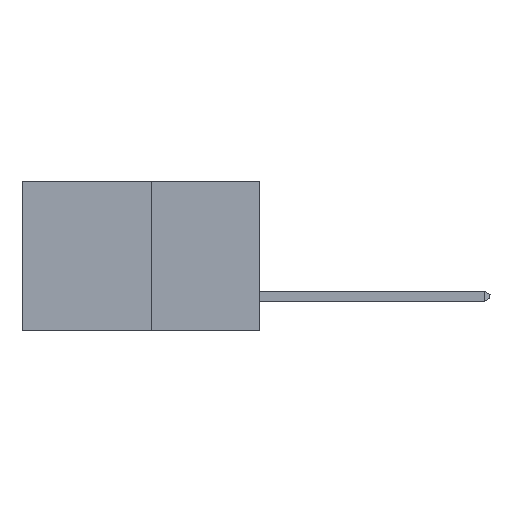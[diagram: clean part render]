
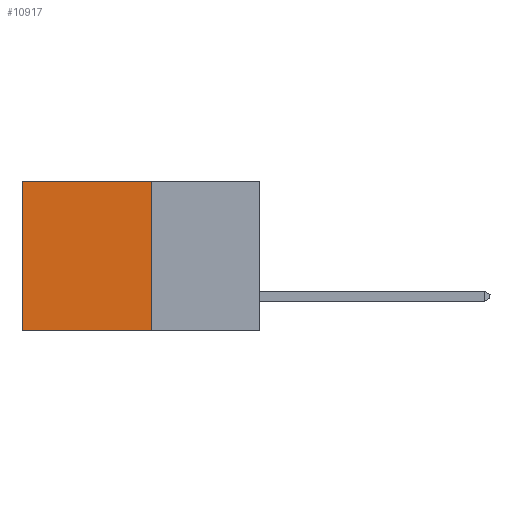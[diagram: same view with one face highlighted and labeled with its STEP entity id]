
A CAD part, left-side view. The second image highlights one B-rep face of the part: STEP entity #10917.
In plain terms, the highlighted planar face has unit normal (-1, 0, 0).
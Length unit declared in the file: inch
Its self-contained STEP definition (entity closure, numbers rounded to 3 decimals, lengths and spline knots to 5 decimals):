
#676 = EDGE_CURVE ( 'NONE', #6583, #10070, #5515, .T. ) ;
#762 = CARTESIAN_POINT ( 'NONE',  ( 0.277, 0.27, 0. ) ) ;
#1182 = DIRECTION ( 'NONE',  ( 0., 0., -1. ) ) ;
#1195 = ORIENTED_EDGE ( 'NONE', *, *, #676, .F. ) ;
#1271 = EDGE_CURVE ( 'NONE', #6583, #7665, #12351, .T. ) ;
#1290 = VECTOR ( 'NONE', #14383, 39.37008 ) ;
#1567 = CARTESIAN_POINT ( 'NONE',  ( 0.277, 0.59, 0. ) ) ;
#1625 = AXIS2_PLACEMENT_3D ( 'NONE', #15243, #8403, #1182 ) ;
#1984 = CARTESIAN_POINT ( 'NONE',  ( 0.277, 0.27, -0.37 ) ) ;
#2161 = LINE ( 'NONE', #12939, #14257 ) ;
#2253 = VECTOR ( 'NONE', #12042, 39.37008 ) ;
#2438 = CARTESIAN_POINT ( 'NONE',  ( 0.277, 0.59, -0.37 ) ) ;
#3572 = CARTESIAN_POINT ( 'NONE',  ( 0.277, 0.27, 0. ) ) ;
#4647 = LINE ( 'NONE', #12113, #1290 ) ;
#4787 = EDGE_LOOP ( 'NONE', ( #7700, #13098, #1195, #12960 ) ) ;
#5515 = LINE ( 'NONE', #14503, #2253 ) ;
#5862 = VECTOR ( 'NONE', #9073, 39.37008 ) ;
#6583 = VERTEX_POINT ( 'NONE', #3572 ) ;
#7665 = VERTEX_POINT ( 'NONE', #1567 ) ;
#7700 = ORIENTED_EDGE ( 'NONE', *, *, #13392, .T. ) ;
#8351 = DIRECTION ( 'NONE',  ( 0., 1., 0. ) ) ;
#8403 = DIRECTION ( 'NONE',  ( 1., 0., 0. ) ) ;
#9073 = DIRECTION ( 'NONE',  ( 0., 1., 0. ) ) ;
#10070 = VERTEX_POINT ( 'NONE', #1984 ) ;
#10861 = FACE_OUTER_BOUND ( 'NONE', #4787, .T. ) ;
#10886 = EDGE_CURVE ( 'NONE', #10070, #13913, #2161, .T. ) ;
#10917 = ADVANCED_FACE ( 'NONE', ( #10861 ), #14143, .F. ) ;
#12042 = DIRECTION ( 'NONE',  ( 0., 0., -1. ) ) ;
#12113 = CARTESIAN_POINT ( 'NONE',  ( 0.277, 0.59, -0.37 ) ) ;
#12351 = LINE ( 'NONE', #762, #5862 ) ;
#12939 = CARTESIAN_POINT ( 'NONE',  ( 0.277, 0.27, -0.37 ) ) ;
#12960 = ORIENTED_EDGE ( 'NONE', *, *, #1271, .T. ) ;
#13098 = ORIENTED_EDGE ( 'NONE', *, *, #10886, .F. ) ;
#13392 = EDGE_CURVE ( 'NONE', #7665, #13913, #4647, .T. ) ;
#13913 = VERTEX_POINT ( 'NONE', #2438 ) ;
#14143 = PLANE ( 'NONE',  #1625 ) ;
#14257 = VECTOR ( 'NONE', #8351, 39.37008 ) ;
#14383 = DIRECTION ( 'NONE',  ( 0., 0., -1. ) ) ;
#14503 = CARTESIAN_POINT ( 'NONE',  ( 0.277, 0.27, -0.37 ) ) ;
#15243 = CARTESIAN_POINT ( 'NONE',  ( 0.277, 0.27, -0.37 ) ) ;
